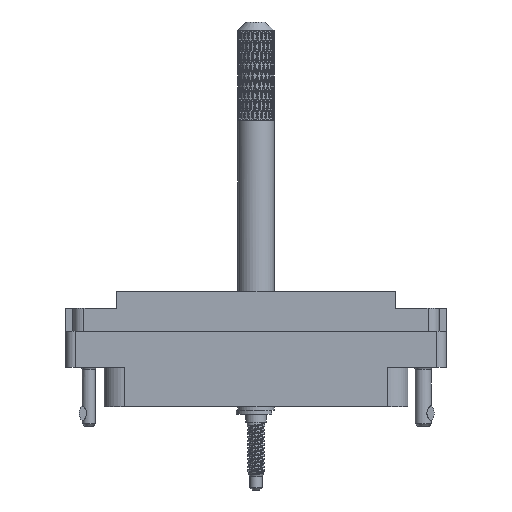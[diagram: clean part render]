
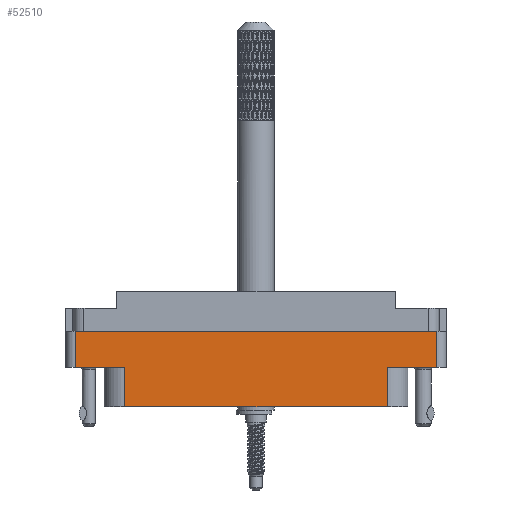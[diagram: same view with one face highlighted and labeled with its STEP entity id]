
A CAD part, front view. The second image highlights one B-rep face of the part: STEP entity #52510.
In plain terms, the highlighted planar face has unit normal (0, -1, 0).
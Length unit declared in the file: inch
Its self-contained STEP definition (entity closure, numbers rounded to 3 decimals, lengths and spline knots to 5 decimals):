
#2922 = CARTESIAN_POINT ( 'NONE',  ( -1.2335, -0.438, -0.789 ) ) ;
#3644 = VECTOR ( 'NONE', #35166, 39.37008 ) ;
#5817 = PLANE ( 'NONE',  #22243 ) ;
#6622 = VERTEX_POINT ( 'NONE', #75321 ) ;
#7192 = VERTEX_POINT ( 'NONE', #33091 ) ;
#9916 = EDGE_CURVE ( 'NONE', #73959, #113451, #44627, .T. ) ;
#12585 = LINE ( 'NONE', #15787, #64737 ) ;
#15178 = DIRECTION ( 'NONE',  ( 0., -1., 0. ) ) ;
#15787 = CARTESIAN_POINT ( 'NONE',  ( 0.895, -0.438, -0.52 ) ) ;
#16325 = CARTESIAN_POINT ( 'NONE',  ( -0.895, -0.438, -0.789 ) ) ;
#17509 = LINE ( 'NONE', #2922, #81306 ) ;
#17724 = CARTESIAN_POINT ( 'NONE',  ( -1.2955, -0.438, -0.789 ) ) ;
#21162 = DIRECTION ( 'NONE',  ( 0., 0., -1. ) ) ;
#22243 = AXIS2_PLACEMENT_3D ( 'NONE', #69851, #15178, #107920 ) ;
#22401 = CARTESIAN_POINT ( 'NONE',  ( 1.2335, -0.438, -0.274 ) ) ;
#25187 = DIRECTION ( 'NONE',  ( 0., 0., -1. ) ) ;
#26172 = DIRECTION ( 'NONE',  ( 1., 0., 0. ) ) ;
#30861 = LINE ( 'NONE', #17724, #101900 ) ;
#31316 = CARTESIAN_POINT ( 'NONE',  ( -1.2335, -0.438, -0.52 ) ) ;
#31829 = CARTESIAN_POINT ( 'NONE',  ( -0.895, -0.438, -0.52 ) ) ;
#32068 = VECTOR ( 'NONE', #25187, 39.37008 ) ;
#32469 = ORIENTED_EDGE ( 'NONE', *, *, #69575, .T. ) ;
#32732 = EDGE_CURVE ( 'NONE', #60208, #6622, #49328, .T. ) ;
#33091 = CARTESIAN_POINT ( 'NONE',  ( -0.895, -0.438, -0.789 ) ) ;
#35166 = DIRECTION ( 'NONE',  ( 0., 0., 1. ) ) ;
#41639 = EDGE_CURVE ( 'NONE', #76678, #7192, #72654, .T. ) ;
#43875 = CARTESIAN_POINT ( 'NONE',  ( 0., -0.438, -0.52 ) ) ;
#44627 = LINE ( 'NONE', #81694, #109905 ) ;
#46410 = DIRECTION ( 'NONE',  ( 1., 0., 0. ) ) ;
#47310 = DIRECTION ( 'NONE',  ( -1., 0., 0. ) ) ;
#49328 = LINE ( 'NONE', #43875, #76874 ) ;
#50209 = ORIENTED_EDGE ( 'NONE', *, *, #32732, .F. ) ;
#52494 = EDGE_LOOP ( 'NONE', ( #75557, #100491, #63523, #85210, #58653, #32469, #50209, #109129 ) ) ;
#52510 = ADVANCED_FACE ( 'NONE', ( #91776 ), #5817, .T. ) ;
#54576 = EDGE_CURVE ( 'NONE', #73959, #97212, #17509, .T. ) ;
#58148 = EDGE_CURVE ( 'NONE', #76678, #97212, #69174, .T. ) ;
#58653 = ORIENTED_EDGE ( 'NONE', *, *, #113128, .T. ) ;
#60208 = VERTEX_POINT ( 'NONE', #65276 ) ;
#61105 = CARTESIAN_POINT ( 'NONE',  ( 1.2335, -0.438, -0.789 ) ) ;
#63523 = ORIENTED_EDGE ( 'NONE', *, *, #58148, .F. ) ;
#64737 = VECTOR ( 'NONE', #107737, 39.37008 ) ;
#65276 = CARTESIAN_POINT ( 'NONE',  ( 1.2335, -0.438, -0.52 ) ) ;
#69174 = LINE ( 'NONE', #85750, #76376 ) ;
#69575 = EDGE_CURVE ( 'NONE', #108967, #6622, #12585, .T. ) ;
#69851 = CARTESIAN_POINT ( 'NONE',  ( -1.2955, -0.438, -0.789 ) ) ;
#71860 = DIRECTION ( 'NONE',  ( -1., 0., 0. ) ) ;
#72654 = LINE ( 'NONE', #16325, #32068 ) ;
#73959 = VERTEX_POINT ( 'NONE', #87596 ) ;
#75321 = CARTESIAN_POINT ( 'NONE',  ( 0.895, -0.438, -0.52 ) ) ;
#75557 = ORIENTED_EDGE ( 'NONE', *, *, #9916, .F. ) ;
#76376 = VECTOR ( 'NONE', #47310, 39.37008 ) ;
#76678 = VERTEX_POINT ( 'NONE', #31829 ) ;
#76874 = VECTOR ( 'NONE', #71860, 39.37008 ) ;
#77273 = CARTESIAN_POINT ( 'NONE',  ( 0.895, -0.438, -0.789 ) ) ;
#81306 = VECTOR ( 'NONE', #21162, 39.37008 ) ;
#81694 = CARTESIAN_POINT ( 'NONE',  ( 0., -0.438, -0.274 ) ) ;
#85210 = ORIENTED_EDGE ( 'NONE', *, *, #41639, .T. ) ;
#85750 = CARTESIAN_POINT ( 'NONE',  ( 0., -0.438, -0.52 ) ) ;
#87596 = CARTESIAN_POINT ( 'NONE',  ( -1.2335, -0.438, -0.274 ) ) ;
#88323 = EDGE_CURVE ( 'NONE', #60208, #113451, #97789, .T. ) ;
#91776 = FACE_OUTER_BOUND ( 'NONE', #52494, .T. ) ;
#97212 = VERTEX_POINT ( 'NONE', #31316 ) ;
#97789 = LINE ( 'NONE', #61105, #3644 ) ;
#100491 = ORIENTED_EDGE ( 'NONE', *, *, #54576, .T. ) ;
#101900 = VECTOR ( 'NONE', #46410, 39.37008 ) ;
#107737 = DIRECTION ( 'NONE',  ( 0., 0., 1. ) ) ;
#107920 = DIRECTION ( 'NONE',  ( 0., 0., -1. ) ) ;
#108967 = VERTEX_POINT ( 'NONE', #77273 ) ;
#109129 = ORIENTED_EDGE ( 'NONE', *, *, #88323, .T. ) ;
#109905 = VECTOR ( 'NONE', #26172, 39.37008 ) ;
#113128 = EDGE_CURVE ( 'NONE', #7192, #108967, #30861, .T. ) ;
#113451 = VERTEX_POINT ( 'NONE', #22401 ) ;
